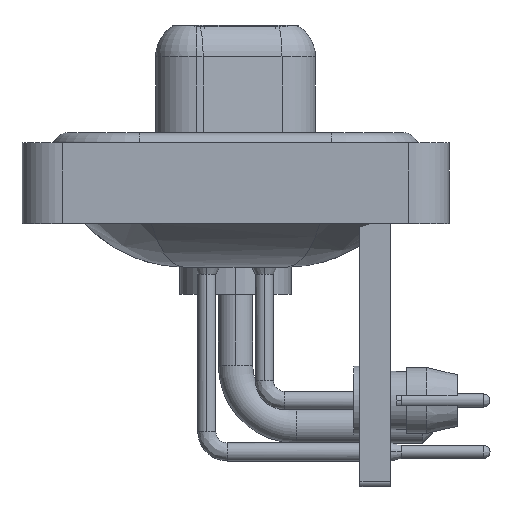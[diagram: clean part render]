
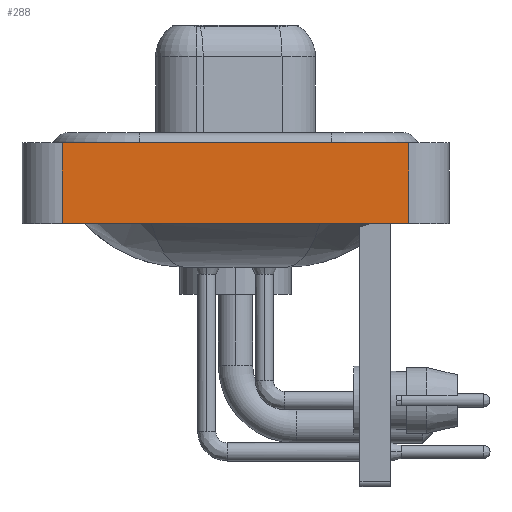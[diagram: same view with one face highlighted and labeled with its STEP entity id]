
A CAD part, left-side view. The second image highlights one B-rep face of the part: STEP entity #288.
In plain terms, the highlighted planar face has unit normal (-1, 0, 0).
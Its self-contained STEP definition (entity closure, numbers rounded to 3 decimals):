
#288 = ADVANCED_FACE ( 'NONE', ( #670 ), #7580, .T. ) ;
#656 = ORIENTED_EDGE ( 'NONE', *, *, #16275, .T. ) ;
#670 = FACE_OUTER_BOUND ( 'NONE', #4530, .T. ) ;
#825 = DIRECTION ( 'NONE',  ( 0., -1., 0. ) ) ;
#1400 = ORIENTED_EDGE ( 'NONE', *, *, #15282, .T. ) ;
#1742 = ORIENTED_EDGE ( 'NONE', *, *, #10759, .F. ) ;
#2665 = DIRECTION ( 'NONE',  ( 0., 0., 1. ) ) ;
#3148 = AXIS2_PLACEMENT_3D ( 'NONE', #7465, #11092, #10990 ) ;
#3467 = CARTESIAN_POINT ( 'NONE',  ( -7.25, 8.55, 0.4 ) ) ;
#3970 = VERTEX_POINT ( 'NONE', #16368 ) ;
#4281 = VERTEX_POINT ( 'NONE', #3467 ) ;
#4401 = VECTOR ( 'NONE', #21652, 1000. ) ;
#4530 = EDGE_LOOP ( 'NONE', ( #656, #14418, #1742, #1400 ) ) ;
#5107 = VECTOR ( 'NONE', #2665, 1000. ) ;
#5133 = EDGE_CURVE ( 'NONE', #4281, #3970, #12827, .T. ) ;
#5846 = CARTESIAN_POINT ( 'NONE',  ( -7.25, 8.55, -3.6 ) ) ;
#5939 = LINE ( 'NONE', #19850, #16357 ) ;
#6250 = CARTESIAN_POINT ( 'NONE',  ( -7.25, -8.55, 0.4 ) ) ;
#7465 = CARTESIAN_POINT ( 'NONE',  ( -7.25, -8.55, -3.6 ) ) ;
#7580 = PLANE ( 'NONE',  #3148 ) ;
#7864 = CARTESIAN_POINT ( 'NONE',  ( -7.25, -8.55, -3.6 ) ) ;
#8874 = VERTEX_POINT ( 'NONE', #7864 ) ;
#10759 = EDGE_CURVE ( 'NONE', #16738, #4281, #10830, .T. ) ;
#10830 = LINE ( 'NONE', #5846, #18440 ) ;
#10990 = DIRECTION ( 'NONE',  ( 0., 0., 1. ) ) ;
#11092 = DIRECTION ( 'NONE',  ( -1., 0., 0. ) ) ;
#12827 = LINE ( 'NONE', #6250, #4401 ) ;
#14418 = ORIENTED_EDGE ( 'NONE', *, *, #5133, .F. ) ;
#15282 = EDGE_CURVE ( 'NONE', #16738, #8874, #5939, .T. ) ;
#16275 = EDGE_CURVE ( 'NONE', #8874, #3970, #16572, .T. ) ;
#16357 = VECTOR ( 'NONE', #825, 1000. ) ;
#16368 = CARTESIAN_POINT ( 'NONE',  ( -7.25, -8.55, 0.4 ) ) ;
#16572 = LINE ( 'NONE', #19879, #5107 ) ;
#16738 = VERTEX_POINT ( 'NONE', #19853 ) ;
#17825 = DIRECTION ( 'NONE',  ( 0., 0., 1. ) ) ;
#18440 = VECTOR ( 'NONE', #17825, 1000. ) ;
#19850 = CARTESIAN_POINT ( 'NONE',  ( -7.25, -8.55, -3.6 ) ) ;
#19853 = CARTESIAN_POINT ( 'NONE',  ( -7.25, 8.55, -3.6 ) ) ;
#19879 = CARTESIAN_POINT ( 'NONE',  ( -7.25, -8.55, -3.6 ) ) ;
#21652 = DIRECTION ( 'NONE',  ( 0., -1., 0. ) ) ;
